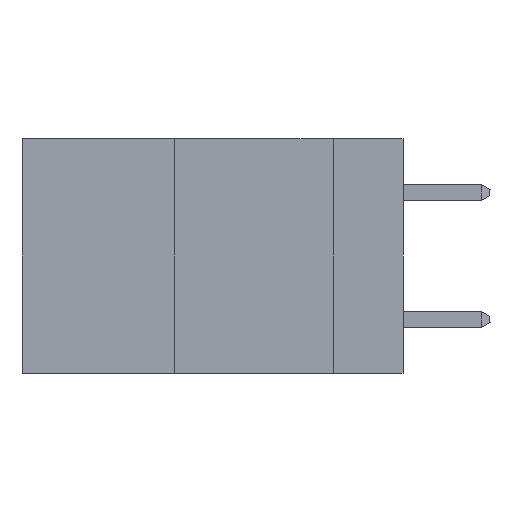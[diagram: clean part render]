
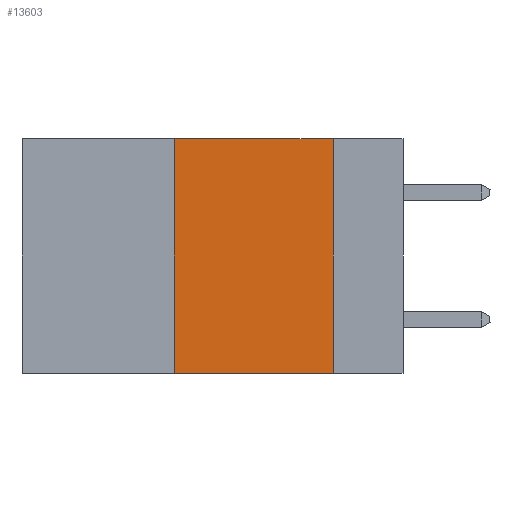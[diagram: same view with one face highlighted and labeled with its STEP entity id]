
A CAD part, left-side view. The second image highlights one B-rep face of the part: STEP entity #13603.
In plain terms, the highlighted planar face has unit normal (-1, 0, 0).
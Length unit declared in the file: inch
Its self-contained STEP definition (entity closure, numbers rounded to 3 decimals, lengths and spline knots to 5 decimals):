
#253 = CARTESIAN_POINT ( 'NONE',  ( 0., 0.36, -0.37 ) ) ;
#379 = CARTESIAN_POINT ( 'NONE',  ( 0., 0.6, 0. ) ) ;
#778 = CARTESIAN_POINT ( 'NONE',  ( 0., 0.6, -0.37 ) ) ;
#854 = EDGE_CURVE ( 'NONE', #17743, #11920, #14363, .T. ) ;
#1277 = DIRECTION ( 'NONE',  ( 0., -1., 0. ) ) ;
#1684 = DIRECTION ( 'NONE',  ( 1., 0., 0. ) ) ;
#2067 = CARTESIAN_POINT ( 'NONE',  ( 0., 0.36, 0. ) ) ;
#2111 = VERTEX_POINT ( 'NONE', #12444 ) ;
#2172 = FACE_OUTER_BOUND ( 'NONE', #11269, .T. ) ;
#2771 = LINE ( 'NONE', #2067, #3853 ) ;
#3313 = DIRECTION ( 'NONE',  ( 0., -1., 0. ) ) ;
#3853 = VECTOR ( 'NONE', #7723, 39.37008 ) ;
#5875 = EDGE_CURVE ( 'NONE', #14834, #2111, #2771, .T. ) ;
#7217 = ORIENTED_EDGE ( 'NONE', *, *, #13887, .T. ) ;
#7723 = DIRECTION ( 'NONE',  ( 0., 0., 1. ) ) ;
#8779 = ORIENTED_EDGE ( 'NONE', *, *, #5875, .F. ) ;
#9690 = LINE ( 'NONE', #778, #12646 ) ;
#10229 = EDGE_CURVE ( 'NONE', #2111, #17743, #13242, .T. ) ;
#10261 = VECTOR ( 'NONE', #3313, 39.37008 ) ;
#10897 = DIRECTION ( 'NONE',  ( 0., 0., -1. ) ) ;
#11269 = EDGE_LOOP ( 'NONE', ( #18305, #12349, #8779, #7217 ) ) ;
#11920 = VERTEX_POINT ( 'NONE', #16749 ) ;
#12349 = ORIENTED_EDGE ( 'NONE', *, *, #10229, .F. ) ;
#12444 = CARTESIAN_POINT ( 'NONE',  ( 0., 0.36, 0. ) ) ;
#12646 = VECTOR ( 'NONE', #1277, 39.37008 ) ;
#13242 = LINE ( 'NONE', #17778, #10261 ) ;
#13381 = DIRECTION ( 'NONE',  ( 0., 0., -1. ) ) ;
#13603 = ADVANCED_FACE ( 'NONE', ( #2172 ), #14908, .F. ) ;
#13797 = CARTESIAN_POINT ( 'NONE',  ( 0., 0.11, 0. ) ) ;
#13887 = EDGE_CURVE ( 'NONE', #14834, #11920, #9690, .T. ) ;
#14363 = LINE ( 'NONE', #13797, #17732 ) ;
#14834 = VERTEX_POINT ( 'NONE', #253 ) ;
#14908 = PLANE ( 'NONE',  #14930 ) ;
#14930 = AXIS2_PLACEMENT_3D ( 'NONE', #379, #1684, #13381 ) ;
#16749 = CARTESIAN_POINT ( 'NONE',  ( 0., 0.11, -0.37 ) ) ;
#17732 = VECTOR ( 'NONE', #10897, 39.37008 ) ;
#17743 = VERTEX_POINT ( 'NONE', #18764 ) ;
#17778 = CARTESIAN_POINT ( 'NONE',  ( 0., 0.6, 0. ) ) ;
#18305 = ORIENTED_EDGE ( 'NONE', *, *, #854, .F. ) ;
#18764 = CARTESIAN_POINT ( 'NONE',  ( 0., 0.11, 0. ) ) ;
